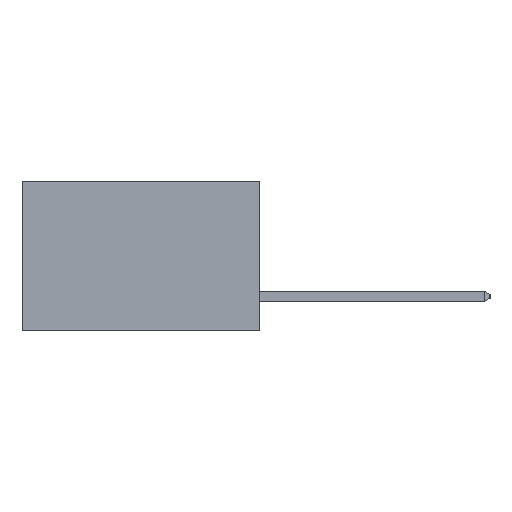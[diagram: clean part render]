
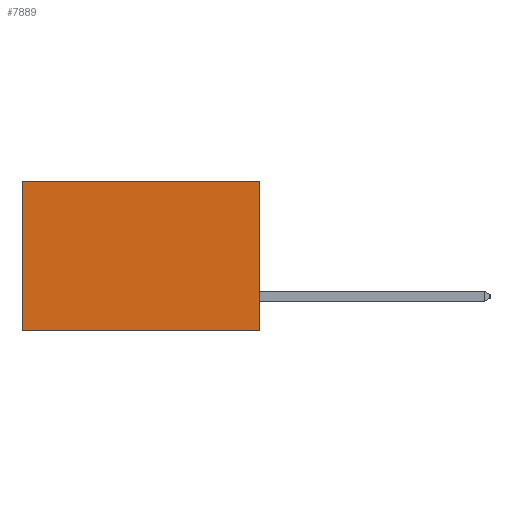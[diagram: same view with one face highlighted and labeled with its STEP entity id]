
A CAD part, left-side view. The second image highlights one B-rep face of the part: STEP entity #7889.
In plain terms, the highlighted planar face has unit normal (-1, 0, 0).
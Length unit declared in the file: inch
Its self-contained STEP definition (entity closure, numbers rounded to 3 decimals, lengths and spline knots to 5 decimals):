
#269 = VERTEX_POINT ( 'NONE', #3985 ) ;
#580 = EDGE_CURVE ( 'NONE', #16732, #6179, #12329, .T. ) ;
#678 = DIRECTION ( 'NONE',  ( 0., 0., -1. ) ) ;
#760 = CARTESIAN_POINT ( 'NONE',  ( 0.277, 0., -0.37 ) ) ;
#956 = ORIENTED_EDGE ( 'NONE', *, *, #580, .T. ) ;
#1275 = DIRECTION ( 'NONE',  ( 0., 1., 0. ) ) ;
#2236 = EDGE_CURVE ( 'NONE', #6179, #14854, #2282, .T. ) ;
#2282 = LINE ( 'NONE', #14656, #2802 ) ;
#2374 = PLANE ( 'NONE',  #20183 ) ;
#2588 = VECTOR ( 'NONE', #9265, 39.37008 ) ;
#2795 = ORIENTED_EDGE ( 'NONE', *, *, #4898, .F. ) ;
#2802 = VECTOR ( 'NONE', #3538, 39.37008 ) ;
#3538 = DIRECTION ( 'NONE',  ( 0., 0., -1. ) ) ;
#3985 = CARTESIAN_POINT ( 'NONE',  ( 0.277, 0., -0.37 ) ) ;
#4027 = CARTESIAN_POINT ( 'NONE',  ( 0.277, 0., -0.37 ) ) ;
#4898 = EDGE_CURVE ( 'NONE', #269, #14854, #10791, .T. ) ;
#5594 = VECTOR ( 'NONE', #678, 39.37008 ) ;
#5703 = DIRECTION ( 'NONE',  ( 0., 0., -1. ) ) ;
#6179 = VERTEX_POINT ( 'NONE', #17184 ) ;
#7494 = EDGE_CURVE ( 'NONE', #16732, #269, #18408, .T. ) ;
#7889 = ADVANCED_FACE ( 'NONE', ( #18391 ), #2374, .F. ) ;
#8535 = EDGE_LOOP ( 'NONE', ( #20430, #2795, #18990, #956 ) ) ;
#9230 = CARTESIAN_POINT ( 'NONE',  ( 0.277, 0.59, -0.37 ) ) ;
#9265 = DIRECTION ( 'NONE',  ( 0., 1., 0. ) ) ;
#9440 = CARTESIAN_POINT ( 'NONE',  ( 0.277, 0., -0.37 ) ) ;
#10791 = LINE ( 'NONE', #9440, #2588 ) ;
#12329 = LINE ( 'NONE', #12746, #20214 ) ;
#12746 = CARTESIAN_POINT ( 'NONE',  ( 0.277, 0., 0. ) ) ;
#14656 = CARTESIAN_POINT ( 'NONE',  ( 0.277, 0.59, -0.37 ) ) ;
#14854 = VERTEX_POINT ( 'NONE', #9230 ) ;
#15356 = DIRECTION ( 'NONE',  ( 1., 0., 0. ) ) ;
#16732 = VERTEX_POINT ( 'NONE', #20570 ) ;
#17184 = CARTESIAN_POINT ( 'NONE',  ( 0.277, 0.59, 0. ) ) ;
#18391 = FACE_OUTER_BOUND ( 'NONE', #8535, .T. ) ;
#18408 = LINE ( 'NONE', #760, #5594 ) ;
#18990 = ORIENTED_EDGE ( 'NONE', *, *, #7494, .F. ) ;
#20183 = AXIS2_PLACEMENT_3D ( 'NONE', #4027, #15356, #5703 ) ;
#20214 = VECTOR ( 'NONE', #1275, 39.37008 ) ;
#20430 = ORIENTED_EDGE ( 'NONE', *, *, #2236, .T. ) ;
#20570 = CARTESIAN_POINT ( 'NONE',  ( 0.277, 0., 0. ) ) ;
